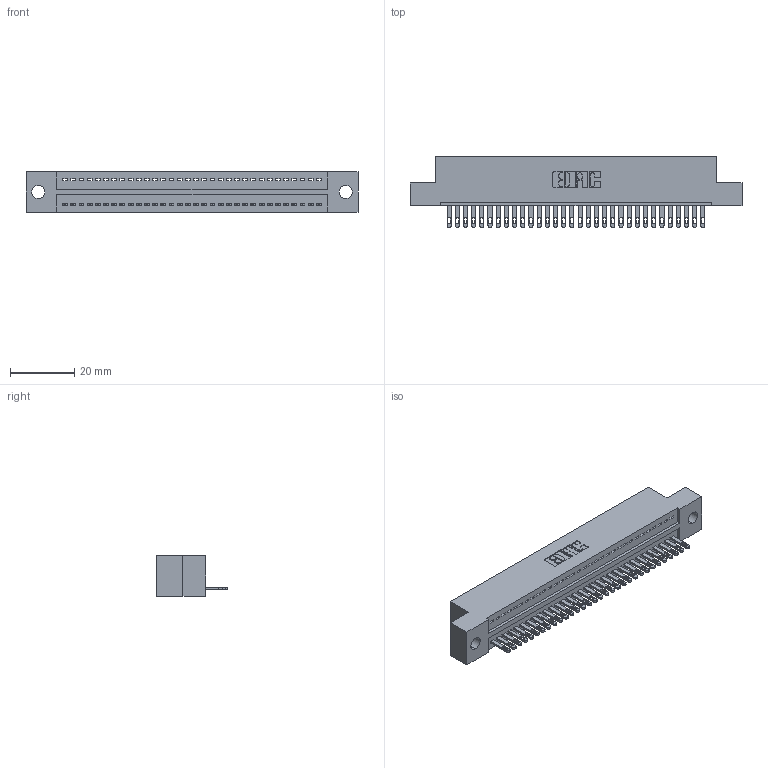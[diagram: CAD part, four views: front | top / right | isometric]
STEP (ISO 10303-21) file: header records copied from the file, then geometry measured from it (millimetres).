
FILE_DESCRIPTION (( 'STEP AP203' ), '1' );
FILE_NAME ('325-032-500-109.STEP', '2020-02-24T19:28:45', ( '' ), ( '' ), 'SwSTEP 2.0', 'SolidWorks 2016', '' );
FILE_SCHEMA (( 'CONFIG_CONTROL_DESIGN' ));
Length unit declared in the file: inch
Products named in the file (3): 325 Part_.160 TH; 325-292-001_325-293-100; 325-032-500-109
Assembly tree (33 placements, depth 2):
  325-032-500-109
    325 Part_.160 TH
    325-292-001_325-293-100  x32
Bounding box: 103 x 21.84 x 12.45 mm (x, y, z)
Volume: 12785.9 mm3; surface area: 13769.6 mm2
Topology: 33 solids, 33 shells, 1842 faces, 5687 edges, 3790 vertices
Faces by surface type: plane 1222, cylinder 620
Entity records: 20789 total; most frequent: CARTESIAN_POINT 3594, ORIENTED_EDGE 3562, DIRECTION 3053, EDGE_CURVE 1781, LINE 1649, VECTOR 1649, VERTEX_POINT 1186, AXIS2_PLACEMENT_3D 702
